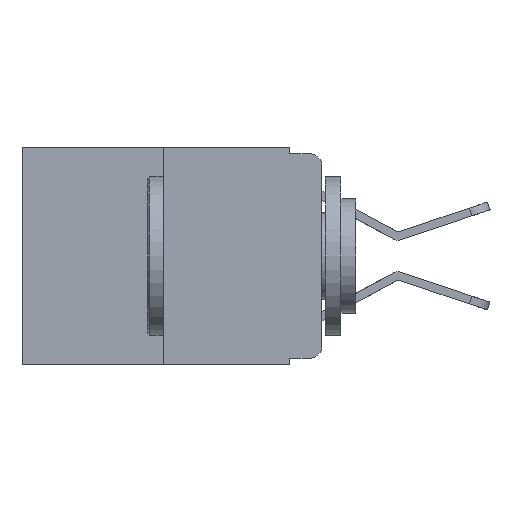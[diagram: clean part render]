
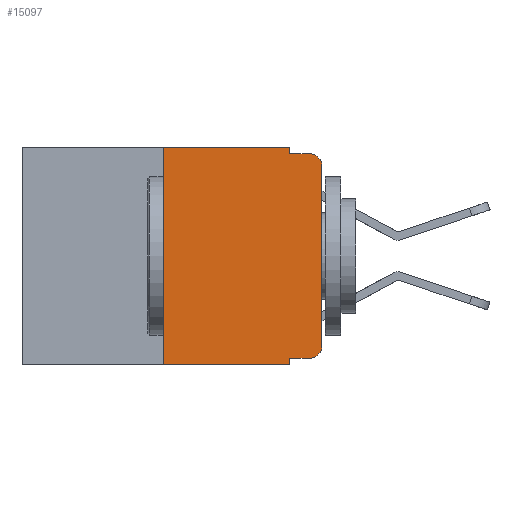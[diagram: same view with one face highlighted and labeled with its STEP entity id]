
A CAD part, left-side view. The second image highlights one B-rep face of the part: STEP entity #15097.
In plain terms, the highlighted planar face has unit normal (-1, 0, 0).
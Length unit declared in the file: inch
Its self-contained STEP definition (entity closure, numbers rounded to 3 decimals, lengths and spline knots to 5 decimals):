
#267 = DIRECTION ( 'NONE',  ( 0., -1., 0. ) ) ;
#379 = CARTESIAN_POINT ( 'NONE',  ( 0., 0.25, -0.343 ) ) ;
#595 = ORIENTED_EDGE ( 'NONE', *, *, #11444, .F. ) ;
#1043 = ORIENTED_EDGE ( 'NONE', *, *, #11706, .F. ) ;
#1124 = CARTESIAN_POINT ( 'NONE',  ( 0., 0., -0.03 ) ) ;
#1383 = CARTESIAN_POINT ( 'NONE',  ( 0., 0.473, 0. ) ) ;
#1971 = DIRECTION ( 'NONE',  ( 0., 0., 1. ) ) ;
#2001 = VECTOR ( 'NONE', #3694, 39.37008 ) ;
#2028 = DIRECTION ( 'NONE',  ( -1., 0., 0. ) ) ;
#2060 = LINE ( 'NONE', #14889, #15651 ) ;
#2117 = EDGE_CURVE ( 'NONE', #10828, #16026, #8051, .T. ) ;
#2256 = VERTEX_POINT ( 'NONE', #379 ) ;
#2397 = VERTEX_POINT ( 'NONE', #16906 ) ;
#2500 = CARTESIAN_POINT ( 'NONE',  ( 0., 0., -0.313 ) ) ;
#2614 = ORIENTED_EDGE ( 'NONE', *, *, #15200, .T. ) ;
#2775 = VERTEX_POINT ( 'NONE', #2778 ) ;
#2778 = CARTESIAN_POINT ( 'NONE',  ( 0., 0.02, -0.01 ) ) ;
#2844 = DIRECTION ( 'NONE',  ( 0., 0., -1. ) ) ;
#2859 = ORIENTED_EDGE ( 'NONE', *, *, #2117, .F. ) ;
#3062 = VERTEX_POINT ( 'NONE', #13525 ) ;
#3167 = DIRECTION ( 'NONE',  ( 0., 0., 1. ) ) ;
#3246 = VECTOR ( 'NONE', #1971, 39.37008 ) ;
#3515 = LINE ( 'NONE', #11071, #16881 ) ;
#3694 = DIRECTION ( 'NONE',  ( 0., -1., 0. ) ) ;
#4078 = VECTOR ( 'NONE', #15721, 39.37008 ) ;
#4658 = CARTESIAN_POINT ( 'NONE',  ( 0., 0.051, -0.343 ) ) ;
#4709 = CIRCLE ( 'NONE', #5943, 0.02 ) ;
#5506 = EDGE_CURVE ( 'NONE', #2256, #16026, #12661, .T. ) ;
#5665 = VERTEX_POINT ( 'NONE', #1124 ) ;
#5943 = AXIS2_PLACEMENT_3D ( 'NONE', #7692, #16549, #8980 ) ;
#6047 = AXIS2_PLACEMENT_3D ( 'NONE', #10133, #2028, #11421 ) ;
#6212 = CARTESIAN_POINT ( 'NONE',  ( 0., 0.25, 0. ) ) ;
#6900 = EDGE_CURVE ( 'NONE', #10828, #2397, #7712, .T. ) ;
#6946 = LINE ( 'NONE', #6212, #3246 ) ;
#7291 = CIRCLE ( 'NONE', #6047, 0.02 ) ;
#7367 = LINE ( 'NONE', #7703, #10363 ) ;
#7512 = FACE_OUTER_BOUND ( 'NONE', #13980, .T. ) ;
#7572 = CARTESIAN_POINT ( 'NONE',  ( 0., 0.051, 0. ) ) ;
#7692 = CARTESIAN_POINT ( 'NONE',  ( 0., 0.02, -0.313 ) ) ;
#7703 = CARTESIAN_POINT ( 'NONE',  ( 0., 0.473, 0. ) ) ;
#7712 = LINE ( 'NONE', #15968, #13706 ) ;
#7886 = EDGE_CURVE ( 'NONE', #5665, #2775, #7291, .T. ) ;
#8051 = LINE ( 'NONE', #15769, #4078 ) ;
#8508 = DIRECTION ( 'NONE',  ( 0., 0., -1. ) ) ;
#8750 = VERTEX_POINT ( 'NONE', #2500 ) ;
#8980 = DIRECTION ( 'NONE',  ( 0., 0., -1. ) ) ;
#8990 = DIRECTION ( 'NONE',  ( 0., -1., 0. ) ) ;
#9167 = EDGE_CURVE ( 'NONE', #2397, #8750, #4709, .T. ) ;
#9686 = DIRECTION ( 'NONE',  ( 0., -1., 0. ) ) ;
#10133 = CARTESIAN_POINT ( 'NONE',  ( 0., 0.02, -0.03 ) ) ;
#10198 = ORIENTED_EDGE ( 'NONE', *, *, #7886, .T. ) ;
#10363 = VECTOR ( 'NONE', #8990, 39.37008 ) ;
#10416 = ORIENTED_EDGE ( 'NONE', *, *, #6900, .T. ) ;
#10811 = PLANE ( 'NONE',  #15494 ) ;
#10828 = VERTEX_POINT ( 'NONE', #15478 ) ;
#10863 = DIRECTION ( 'NONE',  ( 1., 0., 0. ) ) ;
#11071 = CARTESIAN_POINT ( 'NONE',  ( 0., 0.051, -0.01 ) ) ;
#11407 = ORIENTED_EDGE ( 'NONE', *, *, #13554, .F. ) ;
#11421 = DIRECTION ( 'NONE',  ( 0., 0., -1. ) ) ;
#11444 = EDGE_CURVE ( 'NONE', #3062, #2775, #3515, .T. ) ;
#11568 = CARTESIAN_POINT ( 'NONE',  ( 0., 0.473, -0.343 ) ) ;
#11706 = EDGE_CURVE ( 'NONE', #16768, #14438, #7367, .T. ) ;
#11819 = ORIENTED_EDGE ( 'NONE', *, *, #12202, .F. ) ;
#12202 = EDGE_CURVE ( 'NONE', #2256, #16768, #6946, .T. ) ;
#12541 = LINE ( 'NONE', #16079, #15474 ) ;
#12661 = LINE ( 'NONE', #11568, #2001 ) ;
#13525 = CARTESIAN_POINT ( 'NONE',  ( 0., 0.051, -0.01 ) ) ;
#13554 = EDGE_CURVE ( 'NONE', #14438, #3062, #12541, .T. ) ;
#13706 = VECTOR ( 'NONE', #9686, 39.37008 ) ;
#13980 = EDGE_LOOP ( 'NONE', ( #2614, #10198, #595, #11407, #1043, #11819, #15942, #2859, #10416, #14183 ) ) ;
#14183 = ORIENTED_EDGE ( 'NONE', *, *, #9167, .T. ) ;
#14438 = VERTEX_POINT ( 'NONE', #7572 ) ;
#14889 = CARTESIAN_POINT ( 'NONE',  ( 0., 0., 0. ) ) ;
#15097 = ADVANCED_FACE ( 'NONE', ( #7512 ), #10811, .F. ) ;
#15120 = CARTESIAN_POINT ( 'NONE',  ( 0., 0.25, 0. ) ) ;
#15200 = EDGE_CURVE ( 'NONE', #8750, #5665, #2060, .T. ) ;
#15474 = VECTOR ( 'NONE', #8508, 39.37008 ) ;
#15478 = CARTESIAN_POINT ( 'NONE',  ( 0., 0.051, -0.333 ) ) ;
#15494 = AXIS2_PLACEMENT_3D ( 'NONE', #1383, #10863, #2844 ) ;
#15651 = VECTOR ( 'NONE', #3167, 39.37008 ) ;
#15721 = DIRECTION ( 'NONE',  ( 0., 0., -1. ) ) ;
#15769 = CARTESIAN_POINT ( 'NONE',  ( 0., 0.051, 0. ) ) ;
#15942 = ORIENTED_EDGE ( 'NONE', *, *, #5506, .T. ) ;
#15968 = CARTESIAN_POINT ( 'NONE',  ( 0., 0.051, -0.333 ) ) ;
#16026 = VERTEX_POINT ( 'NONE', #4658 ) ;
#16079 = CARTESIAN_POINT ( 'NONE',  ( 0., 0.051, 0. ) ) ;
#16549 = DIRECTION ( 'NONE',  ( -1., 0., 0. ) ) ;
#16768 = VERTEX_POINT ( 'NONE', #15120 ) ;
#16881 = VECTOR ( 'NONE', #267, 39.37008 ) ;
#16906 = CARTESIAN_POINT ( 'NONE',  ( 0., 0.02, -0.333 ) ) ;
